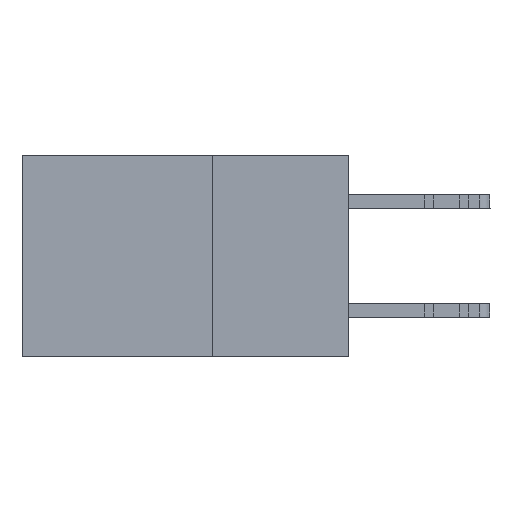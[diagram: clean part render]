
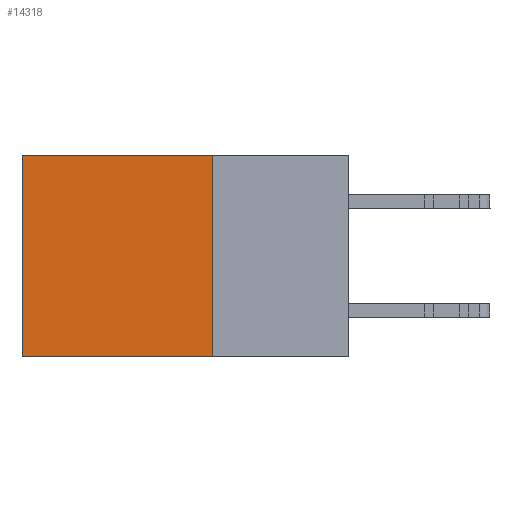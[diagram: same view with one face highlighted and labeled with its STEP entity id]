
A CAD part, left-side view. The second image highlights one B-rep face of the part: STEP entity #14318.
In plain terms, the highlighted planar face has unit normal (-1, 0, 0).
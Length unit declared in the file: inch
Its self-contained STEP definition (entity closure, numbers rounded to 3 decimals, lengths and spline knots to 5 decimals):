
#3275 = EDGE_CURVE ( 'NONE', #19740, #18367, #7965, .T. ) ;
#5245 = PLANE ( 'NONE',  #5391 ) ;
#5288 = ORIENTED_EDGE ( 'NONE', *, *, #15447, .F. ) ;
#5391 = AXIS2_PLACEMENT_3D ( 'NONE', #11083, #12955, #12837 ) ;
#6090 = EDGE_CURVE ( 'NONE', #23026, #13126, #17049, .T. ) ;
#6102 = DIRECTION ( 'NONE',  ( 0., 0., -1. ) ) ;
#6858 = CARTESIAN_POINT ( 'NONE',  ( 0.2615, 0.6, 0. ) ) ;
#7965 = LINE ( 'NONE', #23146, #18987 ) ;
#8607 = VECTOR ( 'NONE', #12426, 39.37008 ) ;
#8745 = ORIENTED_EDGE ( 'NONE', *, *, #6090, .T. ) ;
#9693 = VECTOR ( 'NONE', #17407, 39.37008 ) ;
#9907 = DIRECTION ( 'NONE',  ( 0., 1., 0. ) ) ;
#11063 = CARTESIAN_POINT ( 'NONE',  ( 0.2615, 0.25, -0.37 ) ) ;
#11083 = CARTESIAN_POINT ( 'NONE',  ( 0.2615, 0.25, -0.37 ) ) ;
#11736 = EDGE_LOOP ( 'NONE', ( #8745, #5288, #24359, #17628 ) ) ;
#12426 = DIRECTION ( 'NONE',  ( 0., 1., 0. ) ) ;
#12837 = DIRECTION ( 'NONE',  ( 0., 0., -1. ) ) ;
#12955 = DIRECTION ( 'NONE',  ( 1., 0., 0. ) ) ;
#13126 = VERTEX_POINT ( 'NONE', #21274 ) ;
#14318 = ADVANCED_FACE ( 'NONE', ( #14953 ), #5245, .F. ) ;
#14953 = FACE_OUTER_BOUND ( 'NONE', #11736, .T. ) ;
#15447 = EDGE_CURVE ( 'NONE', #18367, #13126, #16052, .T. ) ;
#15830 = EDGE_CURVE ( 'NONE', #19740, #23026, #19374, .T. ) ;
#16052 = LINE ( 'NONE', #23629, #8607 ) ;
#17049 = LINE ( 'NONE', #23001, #9693 ) ;
#17407 = DIRECTION ( 'NONE',  ( 0., 0., -1. ) ) ;
#17579 = CARTESIAN_POINT ( 'NONE',  ( 0.2615, 0.25, 0. ) ) ;
#17628 = ORIENTED_EDGE ( 'NONE', *, *, #15830, .T. ) ;
#18367 = VERTEX_POINT ( 'NONE', #11063 ) ;
#18987 = VECTOR ( 'NONE', #6102, 39.37008 ) ;
#19374 = LINE ( 'NONE', #22873, #23709 ) ;
#19740 = VERTEX_POINT ( 'NONE', #17579 ) ;
#21274 = CARTESIAN_POINT ( 'NONE',  ( 0.2615, 0.6, -0.37 ) ) ;
#22873 = CARTESIAN_POINT ( 'NONE',  ( 0.2615, 0.25, 0. ) ) ;
#23001 = CARTESIAN_POINT ( 'NONE',  ( 0.2615, 0.6, -0.37 ) ) ;
#23026 = VERTEX_POINT ( 'NONE', #6858 ) ;
#23146 = CARTESIAN_POINT ( 'NONE',  ( 0.2615, 0.25, -0.37 ) ) ;
#23629 = CARTESIAN_POINT ( 'NONE',  ( 0.2615, 0.25, -0.37 ) ) ;
#23709 = VECTOR ( 'NONE', #9907, 39.37008 ) ;
#24359 = ORIENTED_EDGE ( 'NONE', *, *, #3275, .F. ) ;
